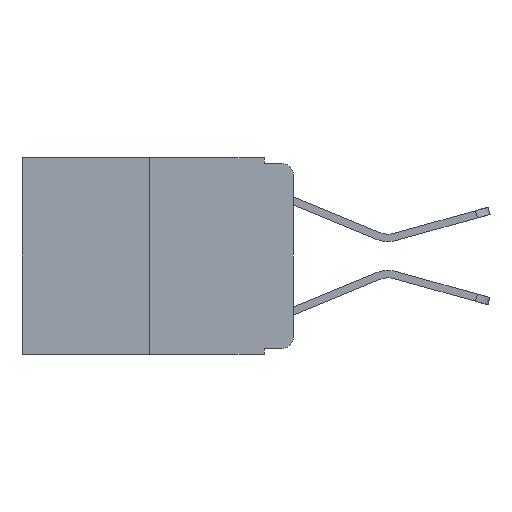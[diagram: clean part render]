
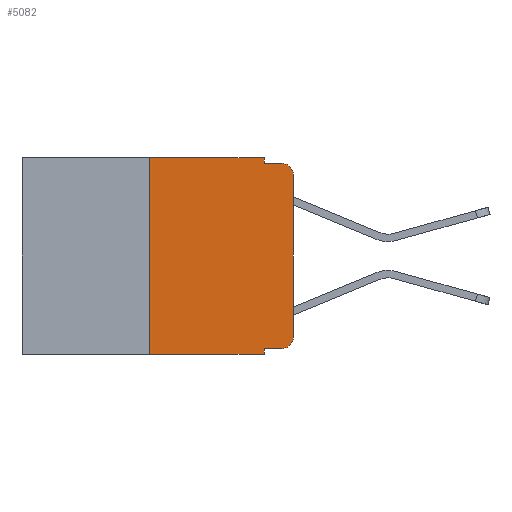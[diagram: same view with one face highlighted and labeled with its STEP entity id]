
A CAD part, left-side view. The second image highlights one B-rep face of the part: STEP entity #5082.
In plain terms, the highlighted planar face has unit normal (-1, 0, 0).
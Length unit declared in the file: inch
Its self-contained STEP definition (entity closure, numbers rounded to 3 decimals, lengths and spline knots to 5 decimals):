
#98 = DIRECTION ( 'NONE',  ( -1., 0., 0. ) ) ;
#181 = ORIENTED_EDGE ( 'NONE', *, *, #1892, .F. ) ;
#333 = ORIENTED_EDGE ( 'NONE', *, *, #9276, .F. ) ;
#382 = VECTOR ( 'NONE', #2365, 39.37008 ) ;
#586 = VERTEX_POINT ( 'NONE', #11210 ) ;
#686 = CARTESIAN_POINT ( 'NONE',  ( 0., 0.051, -0.01 ) ) ;
#740 = ORIENTED_EDGE ( 'NONE', *, *, #3627, .T. ) ;
#931 = CIRCLE ( 'NONE', #7815, 0.02 ) ;
#952 = EDGE_CURVE ( 'NONE', #3375, #8947, #7711, .T. ) ;
#1073 = VERTEX_POINT ( 'NONE', #2598 ) ;
#1172 = LINE ( 'NONE', #11479, #10126 ) ;
#1303 = EDGE_CURVE ( 'NONE', #5846, #5198, #4378, .T. ) ;
#1345 = LINE ( 'NONE', #9610, #8253 ) ;
#1360 = ORIENTED_EDGE ( 'NONE', *, *, #1303, .F. ) ;
#1393 = CARTESIAN_POINT ( 'NONE',  ( 0., 0.051, -0.333 ) ) ;
#1501 = CARTESIAN_POINT ( 'NONE',  ( 0., 0.02, -0.01 ) ) ;
#1772 = VERTEX_POINT ( 'NONE', #5084 ) ;
#1830 = LINE ( 'NONE', #1393, #10928 ) ;
#1892 = EDGE_CURVE ( 'NONE', #11529, #5679, #9986, .T. ) ;
#1926 = VECTOR ( 'NONE', #2550, 39.37008 ) ;
#2280 = DIRECTION ( 'NONE',  ( -1., 0., 0. ) ) ;
#2363 = ORIENTED_EDGE ( 'NONE', *, *, #7050, .T. ) ;
#2365 = DIRECTION ( 'NONE',  ( 0., 0., -1. ) ) ;
#2550 = DIRECTION ( 'NONE',  ( 0., -1., 0. ) ) ;
#2598 = CARTESIAN_POINT ( 'NONE',  ( 0., 0.051, -0.333 ) ) ;
#2640 = ORIENTED_EDGE ( 'NONE', *, *, #10541, .T. ) ;
#2887 = EDGE_CURVE ( 'NONE', #1772, #3375, #7364, .T. ) ;
#3078 = ORIENTED_EDGE ( 'NONE', *, *, #5274, .F. ) ;
#3326 = ORIENTED_EDGE ( 'NONE', *, *, #2887, .T. ) ;
#3375 = VERTEX_POINT ( 'NONE', #10573 ) ;
#3627 = EDGE_CURVE ( 'NONE', #1073, #1772, #1830, .T. ) ;
#3916 = LINE ( 'NONE', #5335, #6300 ) ;
#3956 = CARTESIAN_POINT ( 'NONE',  ( 0., 0.25, -0.343 ) ) ;
#4062 = DIRECTION ( 'NONE',  ( 0., 0., -1. ) ) ;
#4128 = ORIENTED_EDGE ( 'NONE', *, *, #952, .T. ) ;
#4378 = LINE ( 'NONE', #686, #1926 ) ;
#5067 = AXIS2_PLACEMENT_3D ( 'NONE', #7623, #9354, #4062 ) ;
#5082 = ADVANCED_FACE ( 'NONE', ( #6050 ), #6739, .F. ) ;
#5084 = CARTESIAN_POINT ( 'NONE',  ( 0., 0.02, -0.333 ) ) ;
#5198 = VERTEX_POINT ( 'NONE', #1501 ) ;
#5274 = EDGE_CURVE ( 'NONE', #1073, #586, #1345, .T. ) ;
#5303 = LINE ( 'NONE', #7762, #382 ) ;
#5335 = CARTESIAN_POINT ( 'NONE',  ( 0., 0.473, -0.343 ) ) ;
#5488 = DIRECTION ( 'NONE',  ( 0., 0., 1. ) ) ;
#5628 = CARTESIAN_POINT ( 'NONE',  ( 0., 0.02, -0.313 ) ) ;
#5679 = VERTEX_POINT ( 'NONE', #6761 ) ;
#5846 = VERTEX_POINT ( 'NONE', #10436 ) ;
#6050 = FACE_OUTER_BOUND ( 'NONE', #7944, .T. ) ;
#6215 = DIRECTION ( 'NONE',  ( 0., -1., 0. ) ) ;
#6300 = VECTOR ( 'NONE', #6215, 39.37008 ) ;
#6535 = DIRECTION ( 'NONE',  ( 0., 0., -1. ) ) ;
#6679 = EDGE_CURVE ( 'NONE', #8566, #11529, #1172, .T. ) ;
#6739 = PLANE ( 'NONE',  #5067 ) ;
#6761 = CARTESIAN_POINT ( 'NONE',  ( 0., 0.051, 0. ) ) ;
#6917 = ORIENTED_EDGE ( 'NONE', *, *, #6679, .F. ) ;
#7045 = DIRECTION ( 'NONE',  ( 0., 0., -1. ) ) ;
#7050 = EDGE_CURVE ( 'NONE', #8566, #586, #3916, .T. ) ;
#7243 = CARTESIAN_POINT ( 'NONE',  ( 0., 0., 0. ) ) ;
#7348 = CARTESIAN_POINT ( 'NONE',  ( 0., 0., -0.03 ) ) ;
#7364 = CIRCLE ( 'NONE', #8591, 0.02 ) ;
#7623 = CARTESIAN_POINT ( 'NONE',  ( 0., 0.473, 0. ) ) ;
#7680 = CARTESIAN_POINT ( 'NONE',  ( 0., 0.02, -0.03 ) ) ;
#7696 = VECTOR ( 'NONE', #8720, 39.37008 ) ;
#7711 = LINE ( 'NONE', #7243, #10011 ) ;
#7762 = CARTESIAN_POINT ( 'NONE',  ( 0., 0.051, 0. ) ) ;
#7815 = AXIS2_PLACEMENT_3D ( 'NONE', #7680, #2280, #8547 ) ;
#7944 = EDGE_LOOP ( 'NONE', ( #4128, #2640, #1360, #333, #181, #6917, #2363, #3078, #740, #3326 ) ) ;
#8253 = VECTOR ( 'NONE', #7045, 39.37008 ) ;
#8547 = DIRECTION ( 'NONE',  ( 0., 0., -1. ) ) ;
#8566 = VERTEX_POINT ( 'NONE', #3956 ) ;
#8586 = DIRECTION ( 'NONE',  ( 0., -1., 0. ) ) ;
#8591 = AXIS2_PLACEMENT_3D ( 'NONE', #5628, #98, #6535 ) ;
#8720 = DIRECTION ( 'NONE',  ( 0., -1., 0. ) ) ;
#8947 = VERTEX_POINT ( 'NONE', #7348 ) ;
#9276 = EDGE_CURVE ( 'NONE', #5679, #5846, #5303, .T. ) ;
#9354 = DIRECTION ( 'NONE',  ( 1., 0., 0. ) ) ;
#9552 = CARTESIAN_POINT ( 'NONE',  ( 0., 0.473, 0. ) ) ;
#9610 = CARTESIAN_POINT ( 'NONE',  ( 0., 0.051, 0. ) ) ;
#9986 = LINE ( 'NONE', #9552, #7696 ) ;
#10011 = VECTOR ( 'NONE', #10494, 39.37008 ) ;
#10126 = VECTOR ( 'NONE', #5488, 39.37008 ) ;
#10436 = CARTESIAN_POINT ( 'NONE',  ( 0., 0.051, -0.01 ) ) ;
#10494 = DIRECTION ( 'NONE',  ( 0., 0., 1. ) ) ;
#10541 = EDGE_CURVE ( 'NONE', #8947, #5198, #931, .T. ) ;
#10573 = CARTESIAN_POINT ( 'NONE',  ( 0., 0., -0.313 ) ) ;
#10928 = VECTOR ( 'NONE', #8586, 39.37008 ) ;
#11210 = CARTESIAN_POINT ( 'NONE',  ( 0., 0.051, -0.343 ) ) ;
#11479 = CARTESIAN_POINT ( 'NONE',  ( 0., 0.25, 0. ) ) ;
#11515 = CARTESIAN_POINT ( 'NONE',  ( 0., 0.25, 0. ) ) ;
#11529 = VERTEX_POINT ( 'NONE', #11515 ) ;
